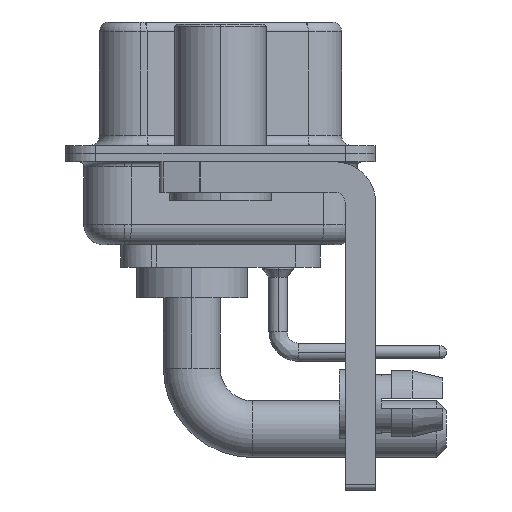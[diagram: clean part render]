
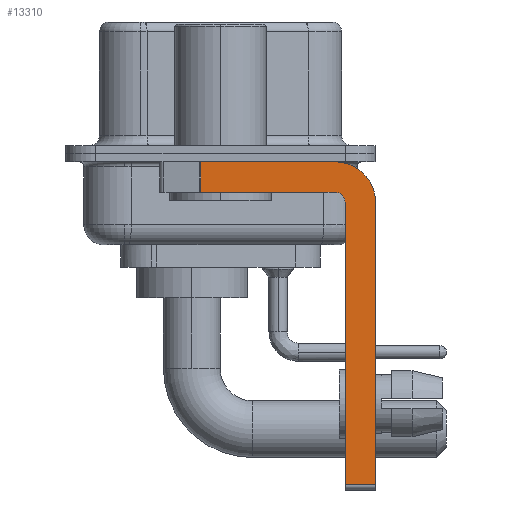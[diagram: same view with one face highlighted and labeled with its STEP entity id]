
A CAD part, left-side view. The second image highlights one B-rep face of the part: STEP entity #13310.
In plain terms, the highlighted planar face has unit normal (-1, 0, 0).
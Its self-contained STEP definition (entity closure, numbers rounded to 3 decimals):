
#483 = ORIENTED_EDGE ( 'NONE', *, *, #16774, .F. ) ;
#1810 = VERTEX_POINT ( 'NONE', #2822 ) ;
#1979 = CARTESIAN_POINT ( 'NONE',  ( -2.9, 0.978, -1.9 ) ) ;
#2227 = DIRECTION ( 'NONE',  ( 1., 0., 0. ) ) ;
#2822 = CARTESIAN_POINT ( 'NONE',  ( -2.9, -7.65, -2.4 ) ) ;
#2852 = VERTEX_POINT ( 'NONE', #3568 ) ;
#3051 = CARTESIAN_POINT ( 'NONE',  ( -2.9, -6.15, -16.6 ) ) ;
#3269 = PLANE ( 'NONE',  #5589 ) ;
#3512 = VERTEX_POINT ( 'NONE', #12998 ) ;
#3568 = CARTESIAN_POINT ( 'NONE',  ( -2.9, -7.65, -16.35 ) ) ;
#4633 = VERTEX_POINT ( 'NONE', #4856 ) ;
#4856 = CARTESIAN_POINT ( 'NONE',  ( -2.9, -6.15, -2.4 ) ) ;
#4921 = DIRECTION ( 'NONE',  ( 0., 1., 0. ) ) ;
#5187 = ORIENTED_EDGE ( 'NONE', *, *, #8533, .F. ) ;
#5251 = ORIENTED_EDGE ( 'NONE', *, *, #8969, .T. ) ;
#5381 = ORIENTED_EDGE ( 'NONE', *, *, #9814, .F. ) ;
#5496 = CARTESIAN_POINT ( 'NONE',  ( -2.9, -5.65, -0.4 ) ) ;
#5589 = AXIS2_PLACEMENT_3D ( 'NONE', #6943, #20261, #15734 ) ;
#5949 = DIRECTION ( 'NONE',  ( -1., 0., 0. ) ) ;
#6055 = EDGE_CURVE ( 'NONE', #19443, #4633, #13949, .T. ) ;
#6258 = VECTOR ( 'NONE', #15572, 1000. ) ;
#6800 = EDGE_CURVE ( 'NONE', #10229, #14555, #14862, .T. ) ;
#6943 = CARTESIAN_POINT ( 'NONE',  ( -2.9, -5.65, -2.4 ) ) ;
#7208 = EDGE_CURVE ( 'NONE', #1810, #2852, #8858, .T. ) ;
#8062 = CIRCLE ( 'NONE', #10272, 0.5 ) ;
#8491 = CARTESIAN_POINT ( 'NONE',  ( -2.9, 3., -0.4 ) ) ;
#8533 = EDGE_CURVE ( 'NONE', #4633, #3512, #8062, .T. ) ;
#8591 = DIRECTION ( 'NONE',  ( 0., 0., -1. ) ) ;
#8858 = LINE ( 'NONE', #26144, #22033 ) ;
#8866 = AXIS2_PLACEMENT_3D ( 'NONE', #23897, #2227, #8591 ) ;
#8969 = EDGE_CURVE ( 'NONE', #19443, #2852, #11522, .T. ) ;
#9682 = DIRECTION ( 'NONE',  ( 0., -1., 0. ) ) ;
#9814 = EDGE_CURVE ( 'NONE', #10229, #18091, #15430, .T. ) ;
#10229 = VERTEX_POINT ( 'NONE', #17385 ) ;
#10272 = AXIS2_PLACEMENT_3D ( 'NONE', #25346, #5949, #14580 ) ;
#10620 = DIRECTION ( 'NONE',  ( 0., 0., -1. ) ) ;
#10643 = CIRCLE ( 'NONE', #8866, 2. ) ;
#11522 = LINE ( 'NONE', #18046, #21585 ) ;
#12096 = DIRECTION ( 'NONE',  ( 0., 0., 1. ) ) ;
#12425 = ORIENTED_EDGE ( 'NONE', *, *, #7208, .F. ) ;
#12998 = CARTESIAN_POINT ( 'NONE',  ( -2.9, -5.65, -1.9 ) ) ;
#13310 = ADVANCED_FACE ( 'NONE', ( #14027 ), #3269, .F. ) ;
#13949 = LINE ( 'NONE', #3051, #21514 ) ;
#14027 = FACE_OUTER_BOUND ( 'NONE', #21704, .T. ) ;
#14555 = VERTEX_POINT ( 'NONE', #17061 ) ;
#14580 = DIRECTION ( 'NONE',  ( 0., 0., 1. ) ) ;
#14683 = DIRECTION ( 'NONE',  ( 0., 0., -1. ) ) ;
#14862 = LINE ( 'NONE', #1979, #17050 ) ;
#14941 = VECTOR ( 'NONE', #4921, 1000. ) ;
#15430 = LINE ( 'NONE', #8491, #6258 ) ;
#15572 = DIRECTION ( 'NONE',  ( 0., -1., 0. ) ) ;
#15734 = DIRECTION ( 'NONE',  ( 0., 0., -1. ) ) ;
#16774 = EDGE_CURVE ( 'NONE', #18091, #1810, #10643, .T. ) ;
#17050 = VECTOR ( 'NONE', #10620, 1000. ) ;
#17061 = CARTESIAN_POINT ( 'NONE',  ( -2.9, 0.978, -1.9 ) ) ;
#17149 = ORIENTED_EDGE ( 'NONE', *, *, #6055, .F. ) ;
#17385 = CARTESIAN_POINT ( 'NONE',  ( -2.9, 0.978, -0.4 ) ) ;
#18046 = CARTESIAN_POINT ( 'NONE',  ( -2.9, -5.65, -16.35 ) ) ;
#18091 = VERTEX_POINT ( 'NONE', #5496 ) ;
#19443 = VERTEX_POINT ( 'NONE', #23192 ) ;
#20261 = DIRECTION ( 'NONE',  ( 1., 0., 0. ) ) ;
#21514 = VECTOR ( 'NONE', #12096, 1000. ) ;
#21585 = VECTOR ( 'NONE', #9682, 1000. ) ;
#21704 = EDGE_LOOP ( 'NONE', ( #5381, #27549, #21830, #5187, #17149, #5251, #12425, #483 ) ) ;
#21830 = ORIENTED_EDGE ( 'NONE', *, *, #27140, .F. ) ;
#22033 = VECTOR ( 'NONE', #14683, 1000. ) ;
#23192 = CARTESIAN_POINT ( 'NONE',  ( -2.9, -6.15, -16.35 ) ) ;
#23897 = CARTESIAN_POINT ( 'NONE',  ( -2.9, -5.65, -2.4 ) ) ;
#24325 = CARTESIAN_POINT ( 'NONE',  ( -2.9, -5.65, -1.9 ) ) ;
#25346 = CARTESIAN_POINT ( 'NONE',  ( -2.9, -5.65, -2.4 ) ) ;
#26144 = CARTESIAN_POINT ( 'NONE',  ( -2.9, -7.65, -2.4 ) ) ;
#26168 = LINE ( 'NONE', #24325, #14941 ) ;
#27140 = EDGE_CURVE ( 'NONE', #3512, #14555, #26168, .T. ) ;
#27549 = ORIENTED_EDGE ( 'NONE', *, *, #6800, .T. ) ;
